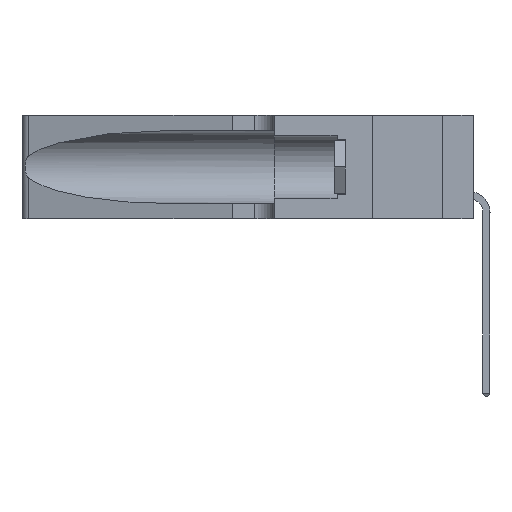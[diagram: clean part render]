
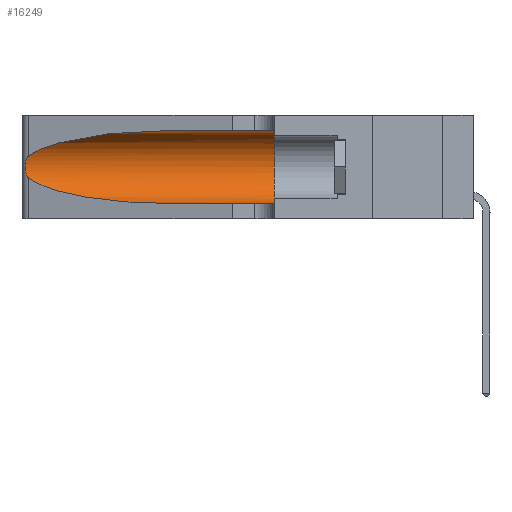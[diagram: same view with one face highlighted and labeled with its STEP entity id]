
A CAD part, left-side view. The second image highlights one B-rep face of the part: STEP entity #16249.
In plain terms, the highlighted cylindrical face has radius 3.308 mm (diameter 6.617 mm), a partial arc.
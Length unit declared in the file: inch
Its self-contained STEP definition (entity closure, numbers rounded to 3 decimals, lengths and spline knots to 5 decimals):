
#36 = ORIENTED_EDGE ( 'NONE', *, *, #5199, .T. ) ;
#123 = EDGE_CURVE ( 'NONE', #4124, #12422, #8283, .T. ) ;
#223 = EDGE_LOOP ( 'NONE', ( #36, #1495, #3082, #11505, #20525, #7111 ) ) ;
#390 = B_SPLINE_CURVE_WITH_KNOTS ( 'NONE', 3,
 ( #11688, #1711, #21787, #13686, #3628, #1635, #9743, #15794, #3722, #1358, #15434, #25479, #17456, #5391 ),
 .UNSPECIFIED., .F., .F.,
 ( 4, 2, 2, 2, 2, 2, 4 ),
 ( 0., 0.00027, 0.00053, 0.00107, 0.0016, 0.00187, 0.00214 ),
 .UNSPECIFIED. ) ;
#1085 = VERTEX_POINT ( 'NONE', #13478 ) ;
#1358 = CARTESIAN_POINT ( 'NONE',  ( 0.25856, 1.23593, 0.16098 ) ) ;
#1495 = ORIENTED_EDGE ( 'NONE', *, *, #18239, .T. ) ;
#1635 = CARTESIAN_POINT ( 'NONE',  ( 0.26018, 1.23835, 0.19895 ) ) ;
#1711 = CARTESIAN_POINT ( 'NONE',  ( 0.25555, 1.22994, 0.2215 ) ) ;
#1971 = CYLINDRICAL_SURFACE ( 'NONE', #22666, 0.13025 ) ;
#2441 = CARTESIAN_POINT ( 'NONE',  ( 0.25487, 1.22718, 0.22369 ) ) ;
#3082 = ORIENTED_EDGE ( 'NONE', *, *, #15745, .T. ) ;
#3323 = LINE ( 'NONE', #6926, #5202 ) ;
#3628 = CARTESIAN_POINT ( 'NONE',  ( 0.25854, 1.2359, 0.20912 ) ) ;
#3722 = CARTESIAN_POINT ( 'NONE',  ( 0.26017, 1.23833, 0.17102 ) ) ;
#3871 = VECTOR ( 'NONE', #22428, 39.37008 ) ;
#3923 = CARTESIAN_POINT ( 'NONE',  ( 0.18966, 0.96281, 0.05475 ) ) ;
#4034 = VERTEX_POINT ( 'NONE', #7580 ) ;
#4124 = VERTEX_POINT ( 'NONE', #21032 ) ;
#4396 = AXIS2_PLACEMENT_3D ( 'NONE', #24588, #20810, #18845 ) ;
#5049 =( BOUNDED_CURVE ( )  B_SPLINE_CURVE ( 3, ( #19317, #9521, #3923, #18088 ),
 .UNSPECIFIED., .F., .F. ) 
 B_SPLINE_CURVE_WITH_KNOTS ( ( 4, 4 ),
 ( 3.44316, 4.71239 ),
 .UNSPECIFIED. ) 
 CURVE ( )  GEOMETRIC_REPRESENTATION_ITEM ( )  RATIONAL_B_SPLINE_CURVE ( ( 1., 0.87, 0.87, 1. ) ) 
 REPRESENTATION_ITEM ( '' )  );
#5199 = EDGE_CURVE ( 'NONE', #4124, #1085, #13637, .T. ) ;
#5202 = VECTOR ( 'NONE', #9140, 39.37008 ) ;
#5391 = CARTESIAN_POINT ( 'NONE',  ( 0.25487, 1.22718, 0.14631 ) ) ;
#5497 = CARTESIAN_POINT ( 'NONE',  ( 0.1305, 0.35, 0.31525 ) ) ;
#5749 = CARTESIAN_POINT ( 'NONE',  ( 0.1305, 1.61858, 0.31525 ) ) ;
#6250 = CIRCLE ( 'NONE', #4396, 0.13025 ) ;
#6926 = CARTESIAN_POINT ( 'NONE',  ( 0.1305, 1.61858, 0.05475 ) ) ;
#7111 = ORIENTED_EDGE ( 'NONE', *, *, #123, .F. ) ;
#7580 = CARTESIAN_POINT ( 'NONE',  ( 0.25487, 1.22718, 0.14631 ) ) ;
#8283 = LINE ( 'NONE', #5749, #3871 ) ;
#8491 = EDGE_CURVE ( 'NONE', #12422, #9801, #6250, .T. ) ;
#9140 = DIRECTION ( 'NONE',  ( 0., -1., 0. ) ) ;
#9521 = CARTESIAN_POINT ( 'NONE',  ( 0.2373, 1.15595, 0.08982 ) ) ;
#9743 = CARTESIAN_POINT ( 'NONE',  ( 0.26075, 1.23896, 0.19203 ) ) ;
#9801 = VERTEX_POINT ( 'NONE', #12991 ) ;
#10419 = EDGE_CURVE ( 'NONE', #15293, #9801, #3323, .T. ) ;
#11074 = CARTESIAN_POINT ( 'NONE',  ( 0.1305, 0.72297, 0.05475 ) ) ;
#11505 = ORIENTED_EDGE ( 'NONE', *, *, #10419, .T. ) ;
#11688 = CARTESIAN_POINT ( 'NONE',  ( 0.25487, 1.22718, 0.22369 ) ) ;
#12422 = VERTEX_POINT ( 'NONE', #5497 ) ;
#12991 = CARTESIAN_POINT ( 'NONE',  ( 0.1305, 0.35, 0.05475 ) ) ;
#13478 = CARTESIAN_POINT ( 'NONE',  ( 0.25487, 1.22718, 0.22369 ) ) ;
#13637 =( BOUNDED_CURVE ( )  B_SPLINE_CURVE ( 3, ( #15911, #22074, #17850, #2441 ),
 .UNSPECIFIED., .F., .F. ) 
 B_SPLINE_CURVE_WITH_KNOTS ( ( 4, 4 ),
 ( 1.5708, 2.84003 ),
 .UNSPECIFIED. ) 
 CURVE ( )  GEOMETRIC_REPRESENTATION_ITEM ( )  RATIONAL_B_SPLINE_CURVE ( ( 1., 0.87, 0.87, 1. ) ) 
 REPRESENTATION_ITEM ( '' )  );
#13686 = CARTESIAN_POINT ( 'NONE',  ( 0.25787, 1.23484, 0.2124 ) ) ;
#14169 = CARTESIAN_POINT ( 'NONE',  ( 0.1305, 1.61858, 0.185 ) ) ;
#14867 = FACE_OUTER_BOUND ( 'NONE', #223, .T. ) ;
#15293 = VERTEX_POINT ( 'NONE', #11074 ) ;
#15434 = CARTESIAN_POINT ( 'NONE',  ( 0.25789, 1.23486, 0.15765 ) ) ;
#15745 = EDGE_CURVE ( 'NONE', #4034, #15293, #5049, .T. ) ;
#15794 = CARTESIAN_POINT ( 'NONE',  ( 0.26075, 1.23896, 0.178 ) ) ;
#15911 = CARTESIAN_POINT ( 'NONE',  ( 0.1305, 0.72297, 0.31525 ) ) ;
#16249 = ADVANCED_FACE ( 'NONE', ( #14867 ), #1971, .F. ) ;
#16347 = DIRECTION ( 'NONE',  ( 0., -1., 0. ) ) ;
#17456 = CARTESIAN_POINT ( 'NONE',  ( 0.25555, 1.22993, 0.14849 ) ) ;
#17850 = CARTESIAN_POINT ( 'NONE',  ( 0.2373, 1.15595, 0.28018 ) ) ;
#18088 = CARTESIAN_POINT ( 'NONE',  ( 0.1305, 0.72297, 0.05475 ) ) ;
#18239 = EDGE_CURVE ( 'NONE', #1085, #4034, #390, .T. ) ;
#18370 = DIRECTION ( 'NONE',  ( 0., 0., -1. ) ) ;
#18845 = DIRECTION ( 'NONE',  ( 0., 0., 1. ) ) ;
#19317 = CARTESIAN_POINT ( 'NONE',  ( 0.25487, 1.22718, 0.14631 ) ) ;
#20525 = ORIENTED_EDGE ( 'NONE', *, *, #8491, .F. ) ;
#20810 = DIRECTION ( 'NONE',  ( 0., 1., 0. ) ) ;
#21032 = CARTESIAN_POINT ( 'NONE',  ( 0.1305, 0.72297, 0.31525 ) ) ;
#21787 = CARTESIAN_POINT ( 'NONE',  ( 0.25639, 1.23184, 0.21858 ) ) ;
#22074 = CARTESIAN_POINT ( 'NONE',  ( 0.18966, 0.96281, 0.31525 ) ) ;
#22428 = DIRECTION ( 'NONE',  ( 0., -1., 0. ) ) ;
#22666 = AXIS2_PLACEMENT_3D ( 'NONE', #14169, #16347, #18370 ) ;
#24588 = CARTESIAN_POINT ( 'NONE',  ( 0.1305, 0.35, 0.185 ) ) ;
#25479 = CARTESIAN_POINT ( 'NONE',  ( 0.25639, 1.23186, 0.15144 ) ) ;
